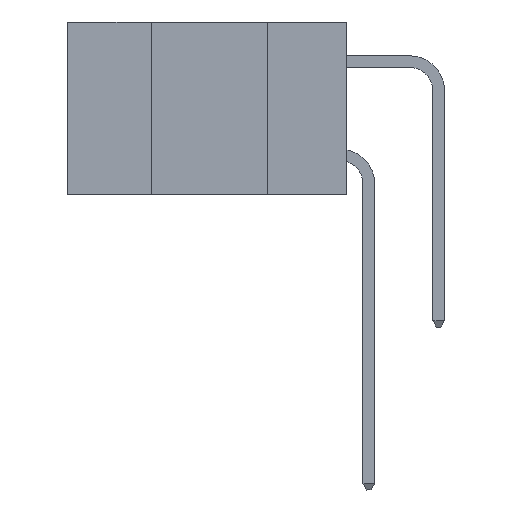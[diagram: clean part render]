
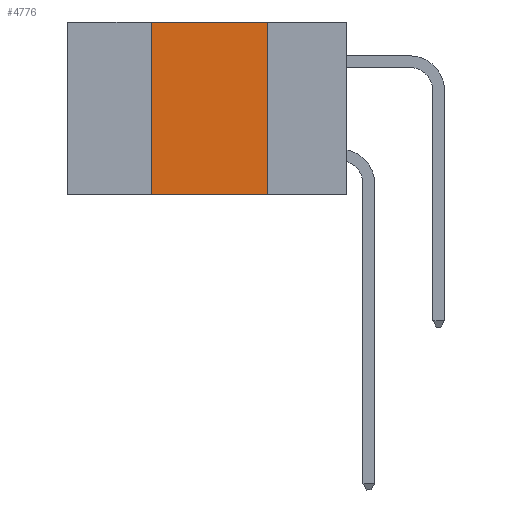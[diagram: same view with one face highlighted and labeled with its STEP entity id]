
A CAD part, left-side view. The second image highlights one B-rep face of the part: STEP entity #4776.
In plain terms, the highlighted planar face has unit normal (-1, 0, 0).
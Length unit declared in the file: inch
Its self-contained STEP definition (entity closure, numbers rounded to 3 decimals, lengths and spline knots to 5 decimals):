
#12 = LINE ( 'NONE', #9524, #20570 ) ;
#1826 = LINE ( 'NONE', #7206, #10473 ) ;
#2050 = DIRECTION ( 'NONE',  ( 0., 0., -1. ) ) ;
#3224 = EDGE_CURVE ( 'NONE', #3455, #13041, #1826, .T. ) ;
#3455 = VERTEX_POINT ( 'NONE', #9238 ) ;
#3831 = VECTOR ( 'NONE', #2050, 39.37008 ) ;
#4226 = CARTESIAN_POINT ( 'NONE',  ( 0., 0.17, 0. ) ) ;
#4370 = EDGE_CURVE ( 'NONE', #3455, #5963, #20632, .T. ) ;
#4776 = ADVANCED_FACE ( 'NONE', ( #9940 ), #14029, .F. ) ;
#5963 = VERTEX_POINT ( 'NONE', #13434 ) ;
#6444 = DIRECTION ( 'NONE',  ( 0., -1., 0. ) ) ;
#6607 = EDGE_CURVE ( 'NONE', #13623, #5963, #20809, .T. ) ;
#7031 = CARTESIAN_POINT ( 'NONE',  ( 0., 0.17, 0. ) ) ;
#7206 = CARTESIAN_POINT ( 'NONE',  ( 0., 0.42, 0. ) ) ;
#7516 = VECTOR ( 'NONE', #8310, 39.37008 ) ;
#7753 = DIRECTION ( 'NONE',  ( 1., 0., 0. ) ) ;
#8310 = DIRECTION ( 'NONE',  ( 0., -1., 0. ) ) ;
#9238 = CARTESIAN_POINT ( 'NONE',  ( 0., 0.42, -0.37 ) ) ;
#9524 = CARTESIAN_POINT ( 'NONE',  ( 0., 0.6, 0. ) ) ;
#9940 = FACE_OUTER_BOUND ( 'NONE', #17610, .T. ) ;
#10473 = VECTOR ( 'NONE', #18261, 39.37008 ) ;
#10561 = ORIENTED_EDGE ( 'NONE', *, *, #6607, .F. ) ;
#13041 = VERTEX_POINT ( 'NONE', #15658 ) ;
#13434 = CARTESIAN_POINT ( 'NONE',  ( 0., 0.17, -0.37 ) ) ;
#13623 = VERTEX_POINT ( 'NONE', #4226 ) ;
#14029 = PLANE ( 'NONE',  #16839 ) ;
#14969 = ORIENTED_EDGE ( 'NONE', *, *, #3224, .F. ) ;
#15658 = CARTESIAN_POINT ( 'NONE',  ( 0., 0.42, 0. ) ) ;
#15980 = ORIENTED_EDGE ( 'NONE', *, *, #20803, .F. ) ;
#16839 = AXIS2_PLACEMENT_3D ( 'NONE', #17243, #7753, #18823 ) ;
#17243 = CARTESIAN_POINT ( 'NONE',  ( 0., 0.6, 0. ) ) ;
#17610 = EDGE_LOOP ( 'NONE', ( #10561, #15980, #14969, #18976 ) ) ;
#18261 = DIRECTION ( 'NONE',  ( 0., 0., 1. ) ) ;
#18823 = DIRECTION ( 'NONE',  ( 0., 0., -1. ) ) ;
#18976 = ORIENTED_EDGE ( 'NONE', *, *, #4370, .T. ) ;
#20570 = VECTOR ( 'NONE', #6444, 39.37008 ) ;
#20632 = LINE ( 'NONE', #20967, #7516 ) ;
#20803 = EDGE_CURVE ( 'NONE', #13041, #13623, #12, .T. ) ;
#20809 = LINE ( 'NONE', #7031, #3831 ) ;
#20967 = CARTESIAN_POINT ( 'NONE',  ( 0., 0.6, -0.37 ) ) ;
